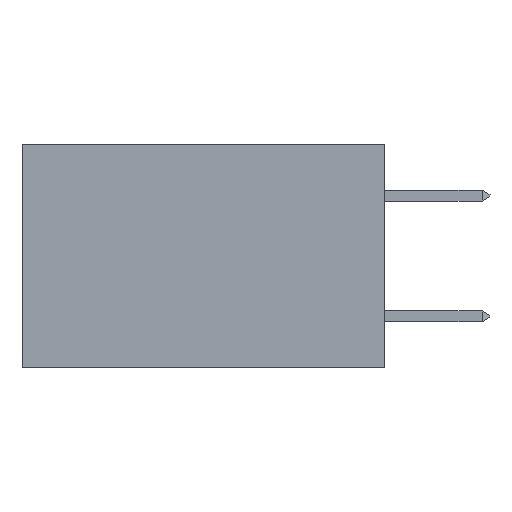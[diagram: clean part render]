
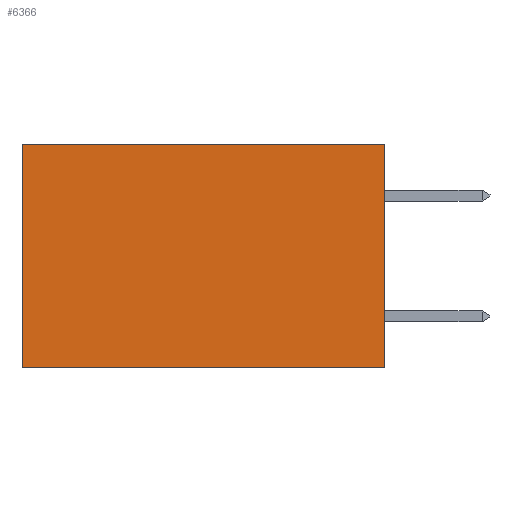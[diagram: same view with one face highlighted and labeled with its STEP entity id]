
A CAD part, left-side view. The second image highlights one B-rep face of the part: STEP entity #6366.
In plain terms, the highlighted planar face has unit normal (-1, 0, 0).
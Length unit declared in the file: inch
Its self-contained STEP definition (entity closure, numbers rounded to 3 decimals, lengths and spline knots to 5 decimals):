
#503 = LINE ( 'NONE', #1712, #5987 ) ;
#1187 = LINE ( 'NONE', #1563, #3454 ) ;
#1563 = CARTESIAN_POINT ( 'NONE',  ( 0.2875, 0., 0. ) ) ;
#1712 = CARTESIAN_POINT ( 'NONE',  ( 0.2875, 0., 0. ) ) ;
#2381 = VECTOR ( 'NONE', #2920, 39.37008 ) ;
#2538 = DIRECTION ( 'NONE',  ( 0., 0., -1. ) ) ;
#2864 = CARTESIAN_POINT ( 'NONE',  ( 0.2875, 0., 0. ) ) ;
#2920 = DIRECTION ( 'NONE',  ( 0., 1., 0. ) ) ;
#3238 = CARTESIAN_POINT ( 'NONE',  ( 0.2875, 0., -0.37 ) ) ;
#3454 = VECTOR ( 'NONE', #2538, 39.37008 ) ;
#3690 = VERTEX_POINT ( 'NONE', #8256 ) ;
#4402 = ORIENTED_EDGE ( 'NONE', *, *, #11054, .T. ) ;
#4473 = DIRECTION ( 'NONE',  ( 0., 0., -1. ) ) ;
#4869 = CARTESIAN_POINT ( 'NONE',  ( 0.2875, 0.6, 0. ) ) ;
#5665 = VERTEX_POINT ( 'NONE', #4869 ) ;
#5909 = LINE ( 'NONE', #6399, #7828 ) ;
#5987 = VECTOR ( 'NONE', #8413, 39.37008 ) ;
#6348 = ORIENTED_EDGE ( 'NONE', *, *, #8690, .F. ) ;
#6366 = ADVANCED_FACE ( 'NONE', ( #9674 ), #8350, .F. ) ;
#6399 = CARTESIAN_POINT ( 'NONE',  ( 0.2875, 0.6, 0. ) ) ;
#7803 = LINE ( 'NONE', #10362, #2381 ) ;
#7828 = VECTOR ( 'NONE', #4473, 39.37008 ) ;
#7923 = VERTEX_POINT ( 'NONE', #3238 ) ;
#7969 = DIRECTION ( 'NONE',  ( 0., 0., -1. ) ) ;
#8070 = EDGE_CURVE ( 'NONE', #5665, #3690, #5909, .T. ) ;
#8162 = DIRECTION ( 'NONE',  ( 1., 0., 0. ) ) ;
#8256 = CARTESIAN_POINT ( 'NONE',  ( 0.2875, 0.6, -0.37 ) ) ;
#8350 = PLANE ( 'NONE',  #8824 ) ;
#8413 = DIRECTION ( 'NONE',  ( 0., 1., 0. ) ) ;
#8548 = ORIENTED_EDGE ( 'NONE', *, *, #8070, .T. ) ;
#8689 = CARTESIAN_POINT ( 'NONE',  ( 0.2875, 0., 0. ) ) ;
#8690 = EDGE_CURVE ( 'NONE', #10594, #7923, #1187, .T. ) ;
#8824 = AXIS2_PLACEMENT_3D ( 'NONE', #8689, #8162, #7969 ) ;
#8945 = EDGE_CURVE ( 'NONE', #7923, #3690, #7803, .T. ) ;
#9674 = FACE_OUTER_BOUND ( 'NONE', #10708, .T. ) ;
#10362 = CARTESIAN_POINT ( 'NONE',  ( 0.2875, 0., -0.37 ) ) ;
#10594 = VERTEX_POINT ( 'NONE', #2864 ) ;
#10708 = EDGE_LOOP ( 'NONE', ( #8548, #10830, #6348, #4402 ) ) ;
#10830 = ORIENTED_EDGE ( 'NONE', *, *, #8945, .F. ) ;
#11054 = EDGE_CURVE ( 'NONE', #10594, #5665, #503, .T. ) ;
